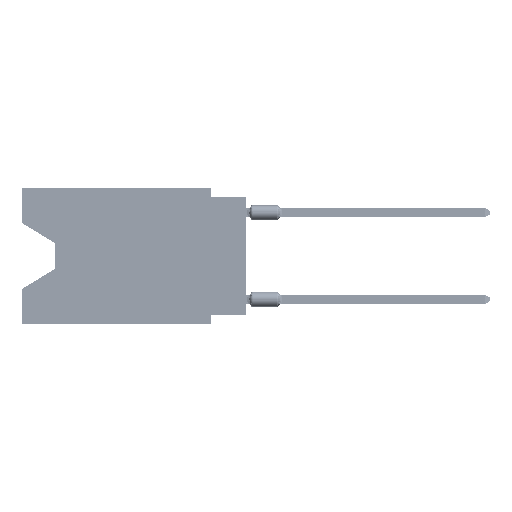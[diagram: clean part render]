
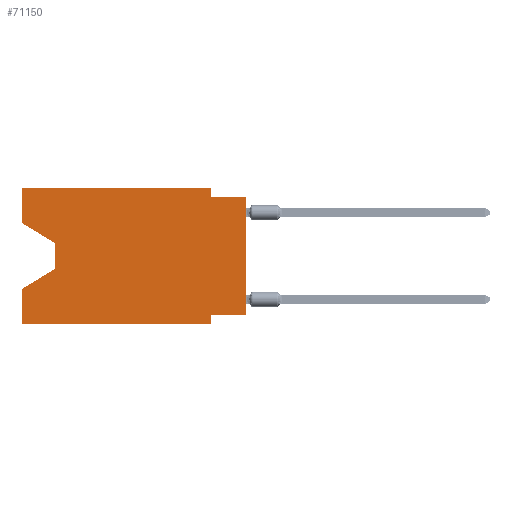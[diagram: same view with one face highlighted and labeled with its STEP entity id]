
A CAD part, left-side view. The second image highlights one B-rep face of the part: STEP entity #71150.
In plain terms, the highlighted planar face has unit normal (-1, 0, 0).
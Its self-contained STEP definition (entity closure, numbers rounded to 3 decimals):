
#76 = VERTEX_POINT ( 'NONE', #29013 ) ;
#1178 = ORIENTED_EDGE ( 'NONE', *, *, #4973, .F. ) ;
#2334 = EDGE_CURVE ( 'NONE', #76, #78385, #34956, .T. ) ;
#3784 = DIRECTION ( 'NONE',  ( 0., -1., 0. ) ) ;
#4973 = EDGE_CURVE ( 'NONE', #61998, #40567, #45801, .T. ) ;
#10138 = CARTESIAN_POINT ( 'NONE',  ( 0., 13.97, -4.013 ) ) ;
#11009 = PLANE ( 'NONE',  #38139 ) ;
#11053 = CARTESIAN_POINT ( 'NONE',  ( 0., 13.97, -5.893 ) ) ;
#15165 = CARTESIAN_POINT ( 'NONE',  ( 0., 13.97, -4.013 ) ) ;
#15637 = DIRECTION ( 'NONE',  ( 0., 0., 1. ) ) ;
#15642 = DIRECTION ( 'NONE',  ( 0., 1., 0. ) ) ;
#16489 = LINE ( 'NONE', #43881, #77270 ) ;
#16636 = VERTEX_POINT ( 'NONE', #82066 ) ;
#16896 = ORIENTED_EDGE ( 'NONE', *, *, #2334, .F. ) ;
#17448 = DIRECTION ( 'NONE',  ( 0., 0., -1. ) ) ;
#18084 = DIRECTION ( 'NONE',  ( 0., 0.855, -0.519 ) ) ;
#18338 = EDGE_CURVE ( 'NONE', #34221, #59802, #85888, .T. ) ;
#21550 = VECTOR ( 'NONE', #41669, 1000. ) ;
#21620 = LINE ( 'NONE', #28798, #41284 ) ;
#23148 = VECTOR ( 'NONE', #18084, 1000. ) ;
#24711 = DIRECTION ( 'NONE',  ( 0., -1., 0. ) ) ;
#24863 = CARTESIAN_POINT ( 'NONE',  ( 0., 16.383, -9.906 ) ) ;
#27473 = CARTESIAN_POINT ( 'NONE',  ( 0., 16.383, 0. ) ) ;
#27664 = VECTOR ( 'NONE', #36778, 1000. ) ;
#27744 = EDGE_CURVE ( 'NONE', #16636, #61998, #83614, .T. ) ;
#28798 = CARTESIAN_POINT ( 'NONE',  ( 0., 0., 0. ) ) ;
#29013 = CARTESIAN_POINT ( 'NONE',  ( 0., 0., -9.271 ) ) ;
#30020 = VECTOR ( 'NONE', #77765, 1000. ) ;
#30035 = LINE ( 'NONE', #72207, #56576 ) ;
#30169 = CARTESIAN_POINT ( 'NONE',  ( 0., 2.54, -9.271 ) ) ;
#30209 = LINE ( 'NONE', #72383, #51358 ) ;
#34221 = VERTEX_POINT ( 'NONE', #85024 ) ;
#34825 = CARTESIAN_POINT ( 'NONE',  ( 0., 2.54, -0.635 ) ) ;
#34956 = LINE ( 'NONE', #55612, #49666 ) ;
#35088 = DIRECTION ( 'NONE',  ( 0., 0., 1. ) ) ;
#36159 = ORIENTED_EDGE ( 'NONE', *, *, #27744, .F. ) ;
#36778 = DIRECTION ( 'NONE',  ( 0., 0., -1. ) ) ;
#38139 = AXIS2_PLACEMENT_3D ( 'NONE', #27473, #74623, #53973 ) ;
#40376 = ORIENTED_EDGE ( 'NONE', *, *, #77974, .T. ) ;
#40567 = VERTEX_POINT ( 'NONE', #48842 ) ;
#40693 = ORIENTED_EDGE ( 'NONE', *, *, #73867, .T. ) ;
#41284 = VECTOR ( 'NONE', #35088, 1000. ) ;
#41669 = DIRECTION ( 'NONE',  ( 0., 0., -1. ) ) ;
#41904 = VECTOR ( 'NONE', #15637, 1000. ) ;
#42226 = ORIENTED_EDGE ( 'NONE', *, *, #87412, .F. ) ;
#43452 = LINE ( 'NONE', #71262, #41904 ) ;
#43516 = LINE ( 'NONE', #70884, #27664 ) ;
#43789 = ORIENTED_EDGE ( 'NONE', *, *, #18338, .T. ) ;
#43881 = CARTESIAN_POINT ( 'NONE',  ( 0., 0., -0.635 ) ) ;
#44137 = DIRECTION ( 'NONE',  ( 0., -0.855, -0.519 ) ) ;
#45801 = LINE ( 'NONE', #79437, #86968 ) ;
#45922 = CARTESIAN_POINT ( 'NONE',  ( 0., 13.97, -5.893 ) ) ;
#47123 = CARTESIAN_POINT ( 'NONE',  ( 0., 0., -0.635 ) ) ;
#48842 = CARTESIAN_POINT ( 'NONE',  ( 0., 2.54, 0. ) ) ;
#49512 = EDGE_CURVE ( 'NONE', #53713, #70576, #77475, .T. ) ;
#49666 = VECTOR ( 'NONE', #15642, 1000. ) ;
#50255 = EDGE_LOOP ( 'NONE', ( #40693, #40376, #56337, #42226, #43789, #75265, #16896, #86041, #87127, #73701, #1178, #36159 ) ) ;
#51358 = VECTOR ( 'NONE', #44137, 1000. ) ;
#52023 = EDGE_CURVE ( 'NONE', #40567, #79572, #30035, .T. ) ;
#53713 = VERTEX_POINT ( 'NONE', #11053 ) ;
#53973 = DIRECTION ( 'NONE',  ( 0., 0., -1. ) ) ;
#55612 = CARTESIAN_POINT ( 'NONE',  ( 0., 0., -9.271 ) ) ;
#56337 = ORIENTED_EDGE ( 'NONE', *, *, #49512, .T. ) ;
#56576 = VECTOR ( 'NONE', #17448, 1000. ) ;
#59802 = VERTEX_POINT ( 'NONE', #83013 ) ;
#59919 = EDGE_CURVE ( 'NONE', #78385, #59802, #43516, .T. ) ;
#61998 = VERTEX_POINT ( 'NONE', #75498 ) ;
#62404 = VERTEX_POINT ( 'NONE', #10138 ) ;
#65773 = FACE_OUTER_BOUND ( 'NONE', #50255, .T. ) ;
#69524 = CARTESIAN_POINT ( 'NONE',  ( 0., 16.383, -7.36 ) ) ;
#70576 = VERTEX_POINT ( 'NONE', #69524 ) ;
#70884 = CARTESIAN_POINT ( 'NONE',  ( 0., 2.54, -9.906 ) ) ;
#71150 = ADVANCED_FACE ( 'NONE', ( #65773 ), #11009, .F. ) ;
#71262 = CARTESIAN_POINT ( 'NONE',  ( 0., 16.383, 0. ) ) ;
#71895 = VECTOR ( 'NONE', #3784, 1000. ) ;
#72207 = CARTESIAN_POINT ( 'NONE',  ( 0., 2.54, 0. ) ) ;
#72383 = CARTESIAN_POINT ( 'NONE',  ( 0., 16.383, -2.546 ) ) ;
#73701 = ORIENTED_EDGE ( 'NONE', *, *, #52023, .F. ) ;
#73867 = EDGE_CURVE ( 'NONE', #16636, #62404, #30209, .T. ) ;
#74623 = DIRECTION ( 'NONE',  ( 1., 0., 0. ) ) ;
#75265 = ORIENTED_EDGE ( 'NONE', *, *, #59919, .F. ) ;
#75477 = EDGE_CURVE ( 'NONE', #76, #85358, #21620, .T. ) ;
#75498 = CARTESIAN_POINT ( 'NONE',  ( 0., 16.383, 0. ) ) ;
#76217 = LINE ( 'NONE', #15165, #21550 ) ;
#77270 = VECTOR ( 'NONE', #83382, 1000. ) ;
#77475 = LINE ( 'NONE', #45922, #23148 ) ;
#77765 = DIRECTION ( 'NONE',  ( 0., 0., 1. ) ) ;
#77974 = EDGE_CURVE ( 'NONE', #62404, #53713, #76217, .T. ) ;
#78385 = VERTEX_POINT ( 'NONE', #30169 ) ;
#79437 = CARTESIAN_POINT ( 'NONE',  ( 0., 16.383, 0. ) ) ;
#79572 = VERTEX_POINT ( 'NONE', #34825 ) ;
#82066 = CARTESIAN_POINT ( 'NONE',  ( 0., 16.383, -2.546 ) ) ;
#83013 = CARTESIAN_POINT ( 'NONE',  ( 0., 2.54, -9.906 ) ) ;
#83251 = EDGE_CURVE ( 'NONE', #79572, #85358, #16489, .T. ) ;
#83382 = DIRECTION ( 'NONE',  ( 0., -1., 0. ) ) ;
#83614 = LINE ( 'NONE', #84493, #30020 ) ;
#84493 = CARTESIAN_POINT ( 'NONE',  ( 0., 16.383, 0. ) ) ;
#85024 = CARTESIAN_POINT ( 'NONE',  ( 0., 16.383, -9.906 ) ) ;
#85358 = VERTEX_POINT ( 'NONE', #47123 ) ;
#85888 = LINE ( 'NONE', #24863, #71895 ) ;
#86041 = ORIENTED_EDGE ( 'NONE', *, *, #75477, .T. ) ;
#86968 = VECTOR ( 'NONE', #24711, 1000. ) ;
#87127 = ORIENTED_EDGE ( 'NONE', *, *, #83251, .F. ) ;
#87412 = EDGE_CURVE ( 'NONE', #34221, #70576, #43452, .T. ) ;
